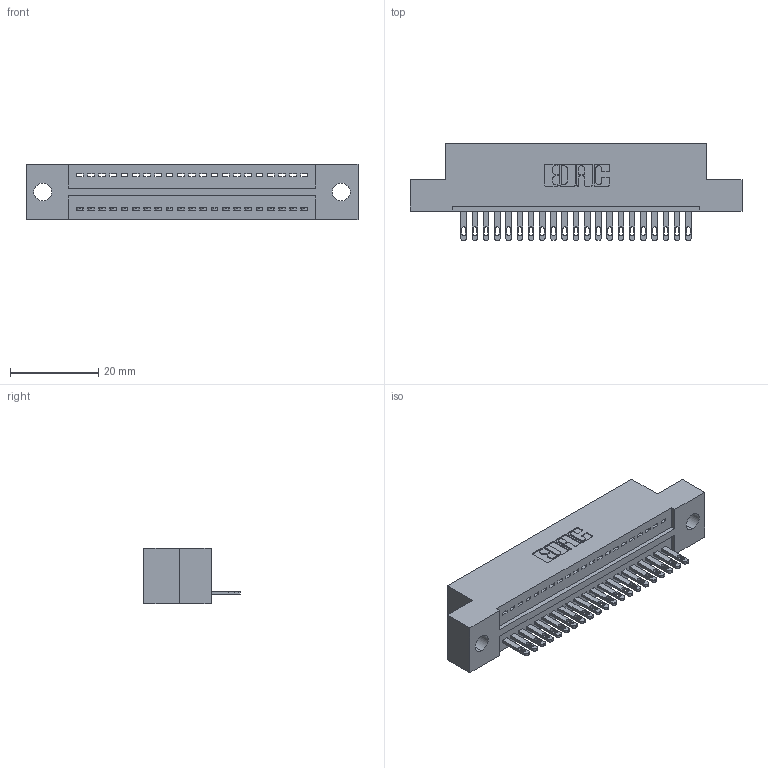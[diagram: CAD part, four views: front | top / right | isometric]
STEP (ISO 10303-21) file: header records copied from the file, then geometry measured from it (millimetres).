
FILE_DESCRIPTION (( 'STEP AP203' ), '1' );
FILE_NAME ('325-021-500-109.STEP', '2020-02-24T17:13:01', ( '' ), ( '' ), 'SwSTEP 2.0', 'SolidWorks 2016', '' );
FILE_SCHEMA (( 'CONFIG_CONTROL_DESIGN' ));
Length unit declared in the file: inch
Products named in the file (3): 325 Part_.160 TH; 325-292-001_325-293-100; 325-021-500-109
Assembly tree (22 placements, depth 2):
  325-021-500-109
    325 Part_.160 TH
    325-292-001_325-293-100  x21
Bounding box: 75.06 x 21.84 x 12.45 mm (x, y, z)
Volume: 9145.6 mm3; surface area: 9580.2 mm2
Topology: 22 solids, 22 shells, 1248 faces, 3839 edges, 2558 vertices
Faces by surface type: plane 826, cylinder 422
Entity records: 15487 total; most frequent: CARTESIAN_POINT 2681, ORIENTED_EDGE 2638, DIRECTION 2305, EDGE_CURVE 1319, LINE 1187, VECTOR 1187, VERTEX_POINT 878, AXIS2_PLACEMENT_3D 559
